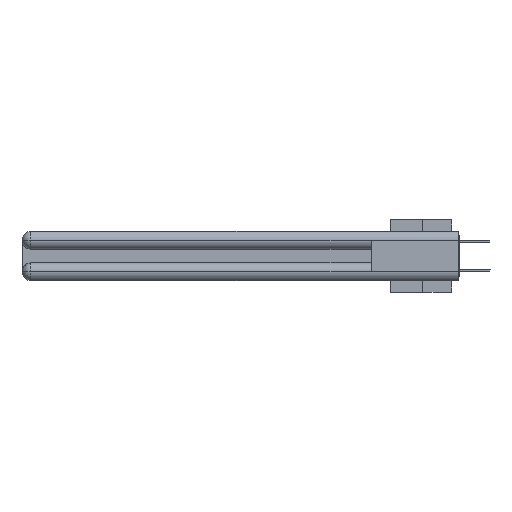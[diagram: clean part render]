
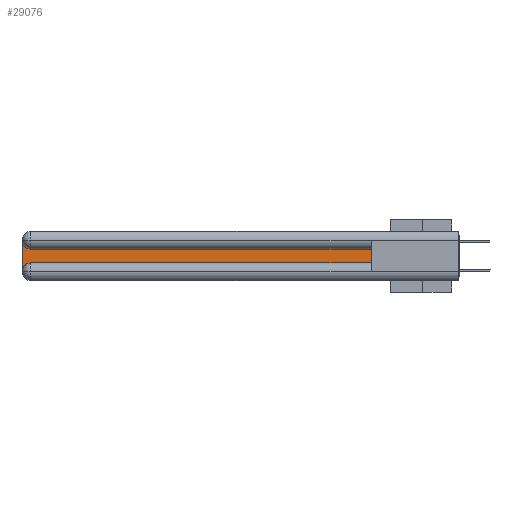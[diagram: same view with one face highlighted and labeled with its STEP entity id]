
A CAD part, left-side view. The second image highlights one B-rep face of the part: STEP entity #29076.
In plain terms, the highlighted planar face has unit normal (-1, 0, 0).
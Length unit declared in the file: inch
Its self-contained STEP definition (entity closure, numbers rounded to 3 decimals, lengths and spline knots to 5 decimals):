
#2487 = DIRECTION ( 'NONE',  ( 0., 0., -1. ) ) ;
#3582 = AXIS2_PLACEMENT_3D ( 'NONE', #13110, #14926, #2487 ) ;
#5218 = LINE ( 'NONE', #30077, #10865 ) ;
#5850 = CARTESIAN_POINT ( 'NONE',  ( 0.075, 3., -0.2775 ) ) ;
#6269 = EDGE_CURVE ( 'NONE', #9554, #10311, #10221, .T. ) ;
#6520 = EDGE_LOOP ( 'NONE', ( #6958, #22613, #15562, #11303, #30523, #24231 ) ) ;
#6630 = CARTESIAN_POINT ( 'NONE',  ( 0.075, 3., -0.1225 ) ) ;
#6895 = VECTOR ( 'NONE', #20628, 39.37008 ) ;
#6958 = ORIENTED_EDGE ( 'NONE', *, *, #26224, .T. ) ;
#7270 = VERTEX_POINT ( 'NONE', #5850 ) ;
#7350 = VERTEX_POINT ( 'NONE', #24324 ) ;
#9403 = DIRECTION ( 'NONE',  ( 0., 0., -1. ) ) ;
#9554 = VERTEX_POINT ( 'NONE', #26071 ) ;
#10221 = LINE ( 'NONE', #12526, #27879 ) ;
#10311 = VERTEX_POINT ( 'NONE', #12022 ) ;
#10865 = VECTOR ( 'NONE', #15195, 39.37008 ) ;
#10887 = CIRCLE ( 'NONE', #21345, 0.06 ) ;
#11303 = ORIENTED_EDGE ( 'NONE', *, *, #19334, .T. ) ;
#11535 = DIRECTION ( 'NONE',  ( 1., 0., 0. ) ) ;
#11622 = EDGE_CURVE ( 'NONE', #10311, #7350, #30101, .T. ) ;
#11711 = CARTESIAN_POINT ( 'NONE',  ( 0.075, 2.94, -0.1225 ) ) ;
#12022 = CARTESIAN_POINT ( 'NONE',  ( 0.075, 0.6, -0.2175 ) ) ;
#12526 = CARTESIAN_POINT ( 'NONE',  ( 0.075, 0.6, -0.2175 ) ) ;
#13110 = CARTESIAN_POINT ( 'NONE',  ( 0.075, 2.94, -0.0625 ) ) ;
#13397 = CARTESIAN_POINT ( 'NONE',  ( 0.075, 0.6, -0.2175 ) ) ;
#14926 = DIRECTION ( 'NONE',  ( 1., 0., 0. ) ) ;
#14992 = VECTOR ( 'NONE', #19736, 39.37008 ) ;
#15195 = DIRECTION ( 'NONE',  ( 0., 0., -1. ) ) ;
#15562 = ORIENTED_EDGE ( 'NONE', *, *, #17514, .T. ) ;
#17107 = LINE ( 'NONE', #26775, #14992 ) ;
#17514 = EDGE_CURVE ( 'NONE', #27752, #7270, #5218, .T. ) ;
#18811 = AXIS2_PLACEMENT_3D ( 'NONE', #6630, #11535, #9403 ) ;
#19334 = EDGE_CURVE ( 'NONE', #7270, #9554, #10887, .T. ) ;
#19736 = DIRECTION ( 'NONE',  ( 0., 1., 0. ) ) ;
#20216 = DIRECTION ( 'NONE',  ( 0., -1., 0. ) ) ;
#20628 = DIRECTION ( 'NONE',  ( 0., 0., 1. ) ) ;
#21345 = AXIS2_PLACEMENT_3D ( 'NONE', #24572, #24407, #30397 ) ;
#21354 = CIRCLE ( 'NONE', #3582, 0.06 ) ;
#22613 = ORIENTED_EDGE ( 'NONE', *, *, #27924, .T. ) ;
#24231 = ORIENTED_EDGE ( 'NONE', *, *, #11622, .T. ) ;
#24324 = CARTESIAN_POINT ( 'NONE',  ( 0.075, 0.6, -0.1225 ) ) ;
#24407 = DIRECTION ( 'NONE',  ( 1., 0., 0. ) ) ;
#24572 = CARTESIAN_POINT ( 'NONE',  ( 0.075, 2.94, -0.2775 ) ) ;
#26071 = CARTESIAN_POINT ( 'NONE',  ( 0.075, 2.94, -0.2175 ) ) ;
#26224 = EDGE_CURVE ( 'NONE', #7350, #31776, #17107, .T. ) ;
#26775 = CARTESIAN_POINT ( 'NONE',  ( 0.075, 0.6, -0.1225 ) ) ;
#27752 = VERTEX_POINT ( 'NONE', #31923 ) ;
#27879 = VECTOR ( 'NONE', #20216, 39.37008 ) ;
#27924 = EDGE_CURVE ( 'NONE', #31776, #27752, #21354, .T. ) ;
#29050 = FACE_OUTER_BOUND ( 'NONE', #6520, .T. ) ;
#29076 = ADVANCED_FACE ( 'NONE', ( #29050 ), #29208, .F. ) ;
#29208 = PLANE ( 'NONE',  #18811 ) ;
#30077 = CARTESIAN_POINT ( 'NONE',  ( 0.075, 3., -0.2175 ) ) ;
#30101 = LINE ( 'NONE', #13397, #6895 ) ;
#30397 = DIRECTION ( 'NONE',  ( 0., 0., -1. ) ) ;
#30523 = ORIENTED_EDGE ( 'NONE', *, *, #6269, .T. ) ;
#31776 = VERTEX_POINT ( 'NONE', #11711 ) ;
#31923 = CARTESIAN_POINT ( 'NONE',  ( 0.075, 3., -0.0625 ) ) ;
